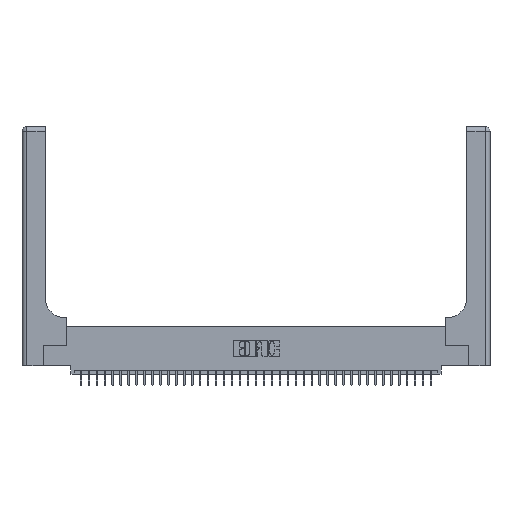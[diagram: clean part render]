
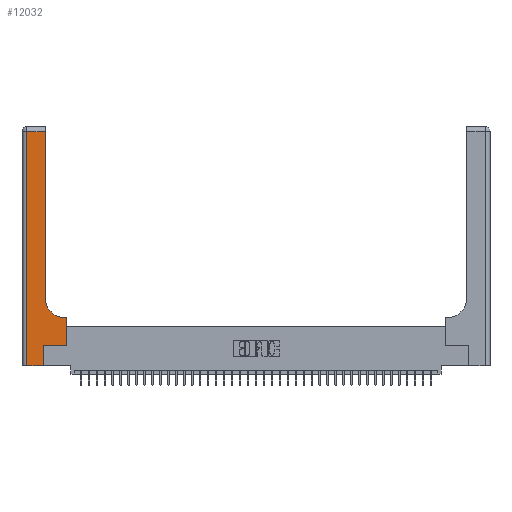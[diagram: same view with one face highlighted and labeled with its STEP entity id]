
A CAD part, top view. The second image highlights one B-rep face of the part: STEP entity #12032.
In plain terms, the highlighted planar face has unit normal (0, 0, 1).
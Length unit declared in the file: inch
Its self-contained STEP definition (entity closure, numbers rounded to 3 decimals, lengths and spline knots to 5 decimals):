
#446 = VERTEX_POINT ( 'NONE', #12172 ) ;
#1932 = CARTESIAN_POINT ( 'NONE',  ( 0.06, 2.94, 0.37 ) ) ;
#2055 = VECTOR ( 'NONE', #5310, 39.37008 ) ;
#2095 = LINE ( 'NONE', #16988, #37336 ) ;
#2932 = EDGE_CURVE ( 'NONE', #27422, #9580, #21003, .T. ) ;
#3060 = VERTEX_POINT ( 'NONE', #28362 ) ;
#3360 = DIRECTION ( 'NONE',  ( 1., 0., 0. ) ) ;
#4035 = CARTESIAN_POINT ( 'NONE',  ( 0.06, 3., 0.37 ) ) ;
#4312 = VECTOR ( 'NONE', #9089, 39.37008 ) ;
#4901 = VECTOR ( 'NONE', #22947, 39.37008 ) ;
#5107 = CARTESIAN_POINT ( 'NONE',  ( 0.5585, 0.6, 0.37 ) ) ;
#5310 = DIRECTION ( 'NONE',  ( 1., 0., 0. ) ) ;
#6398 = EDGE_CURVE ( 'NONE', #13062, #13340, #15637, .T. ) ;
#6452 = ORIENTED_EDGE ( 'NONE', *, *, #2932, .T. ) ;
#6807 = CARTESIAN_POINT ( 'NONE',  ( 0.269, 0.25, 0.37 ) ) ;
#6872 = ORIENTED_EDGE ( 'NONE', *, *, #30826, .T. ) ;
#7325 = DIRECTION ( 'NONE',  ( -1., 0., 0. ) ) ;
#7494 = EDGE_CURVE ( 'NONE', #26863, #446, #35319, .T. ) ;
#8521 = ORIENTED_EDGE ( 'NONE', *, *, #7494, .T. ) ;
#8974 = VERTEX_POINT ( 'NONE', #21909 ) ;
#9089 = DIRECTION ( 'NONE',  ( -1., 0., 0. ) ) ;
#9229 = VECTOR ( 'NONE', #17154, 39.37008 ) ;
#9580 = VERTEX_POINT ( 'NONE', #23475 ) ;
#10716 = LINE ( 'NONE', #15693, #4901 ) ;
#10951 = ORIENTED_EDGE ( 'NONE', *, *, #19546, .T. ) ;
#11006 = DIRECTION ( 'NONE',  ( 1., 0., 0. ) ) ;
#11051 = EDGE_CURVE ( 'NONE', #446, #32690, #32239, .T. ) ;
#11518 = PLANE ( 'NONE',  #36880 ) ;
#12032 = ADVANCED_FACE ( 'NONE', ( #39478 ), #11518, .F. ) ;
#12172 = CARTESIAN_POINT ( 'NONE',  ( 0.2915, 2.94, 0.37 ) ) ;
#12836 = CARTESIAN_POINT ( 'NONE',  ( 0.5415, 0.6, 0.37 ) ) ;
#13062 = VERTEX_POINT ( 'NONE', #5107 ) ;
#13322 = EDGE_CURVE ( 'NONE', #9580, #8974, #10716, .T. ) ;
#13340 = VERTEX_POINT ( 'NONE', #12836 ) ;
#13631 = ORIENTED_EDGE ( 'NONE', *, *, #32330, .T. ) ;
#13962 = CARTESIAN_POINT ( 'NONE',  ( 0., 3., 0.37 ) ) ;
#14629 = CARTESIAN_POINT ( 'NONE',  ( 0.2915, 0.85, 0.37 ) ) ;
#15637 = LINE ( 'NONE', #40126, #4312 ) ;
#15693 = CARTESIAN_POINT ( 'NONE',  ( 0.269, 0., 0.37 ) ) ;
#16232 = ORIENTED_EDGE ( 'NONE', *, *, #34230, .T. ) ;
#16539 = CARTESIAN_POINT ( 'NONE',  ( 0.2915, 3., 0.37 ) ) ;
#16988 = CARTESIAN_POINT ( 'NONE',  ( 0.5585, 0.25, 0.37 ) ) ;
#17154 = DIRECTION ( 'NONE',  ( 0., 1., 0. ) ) ;
#17943 = ORIENTED_EDGE ( 'NONE', *, *, #13322, .T. ) ;
#18706 = EDGE_LOOP ( 'NONE', ( #8521, #23418, #6872, #6452, #17943, #10951, #16232, #27602, #13631 ) ) ;
#19320 = DIRECTION ( 'NONE',  ( 0., -1., 0. ) ) ;
#19432 = CARTESIAN_POINT ( 'NONE',  ( 0.06, 0., 0.37 ) ) ;
#19546 = EDGE_CURVE ( 'NONE', #8974, #3060, #28863, .T. ) ;
#20382 = CARTESIAN_POINT ( 'NONE',  ( 0.5415, 0.85, 0.37 ) ) ;
#21003 = LINE ( 'NONE', #33476, #2055 ) ;
#21909 = CARTESIAN_POINT ( 'NONE',  ( 0.269, 0.25, 0.37 ) ) ;
#22947 = DIRECTION ( 'NONE',  ( 0., 1., 0. ) ) ;
#23418 = ORIENTED_EDGE ( 'NONE', *, *, #11051, .T. ) ;
#23475 = CARTESIAN_POINT ( 'NONE',  ( 0.269, 0., 0.37 ) ) ;
#25427 = VECTOR ( 'NONE', #3360, 39.37008 ) ;
#25440 = VECTOR ( 'NONE', #19320, 39.37008 ) ;
#25721 = VECTOR ( 'NONE', #7325, 39.37008 ) ;
#26520 = DIRECTION ( 'NONE',  ( 0., 0., -1. ) ) ;
#26863 = VERTEX_POINT ( 'NONE', #14629 ) ;
#27422 = VERTEX_POINT ( 'NONE', #19432 ) ;
#27602 = ORIENTED_EDGE ( 'NONE', *, *, #6398, .T. ) ;
#28362 = CARTESIAN_POINT ( 'NONE',  ( 0.5585, 0.25, 0.37 ) ) ;
#28863 = LINE ( 'NONE', #6807, #25427 ) ;
#30826 = EDGE_CURVE ( 'NONE', #32690, #27422, #31987, .T. ) ;
#31987 = LINE ( 'NONE', #4035, #25440 ) ;
#32239 = LINE ( 'NONE', #35499, #25721 ) ;
#32330 = EDGE_CURVE ( 'NONE', #13340, #26863, #33345, .T. ) ;
#32690 = VERTEX_POINT ( 'NONE', #1932 ) ;
#32905 = DIRECTION ( 'NONE',  ( 0., 1., 0. ) ) ;
#33147 = DIRECTION ( 'NONE',  ( 0., 0., -1. ) ) ;
#33345 = CIRCLE ( 'NONE', #36514, 0.25 ) ;
#33476 = CARTESIAN_POINT ( 'NONE',  ( 0., 0., 0.37 ) ) ;
#34230 = EDGE_CURVE ( 'NONE', #3060, #13062, #2095, .T. ) ;
#35319 = LINE ( 'NONE', #16539, #9229 ) ;
#35499 = CARTESIAN_POINT ( 'NONE',  ( 0., 2.94, 0.37 ) ) ;
#36514 = AXIS2_PLACEMENT_3D ( 'NONE', #20382, #26520, #11006 ) ;
#36880 = AXIS2_PLACEMENT_3D ( 'NONE', #13962, #33147, #38858 ) ;
#37336 = VECTOR ( 'NONE', #32905, 39.37008 ) ;
#38858 = DIRECTION ( 'NONE',  ( -1., 0., 0. ) ) ;
#39478 = FACE_OUTER_BOUND ( 'NONE', #18706, .T. ) ;
#40126 = CARTESIAN_POINT ( 'NONE',  ( 0.2915, 0.6, 0.37 ) ) ;
